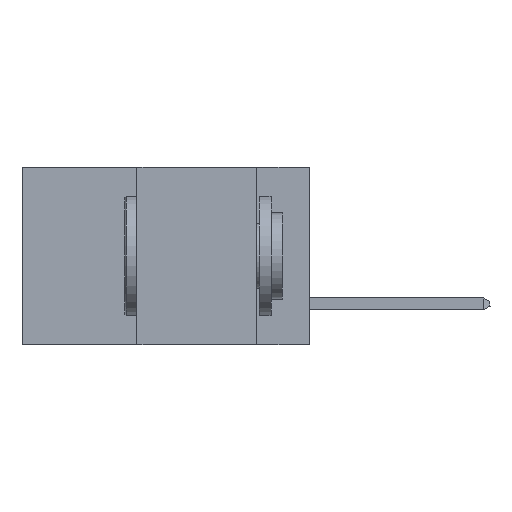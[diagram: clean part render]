
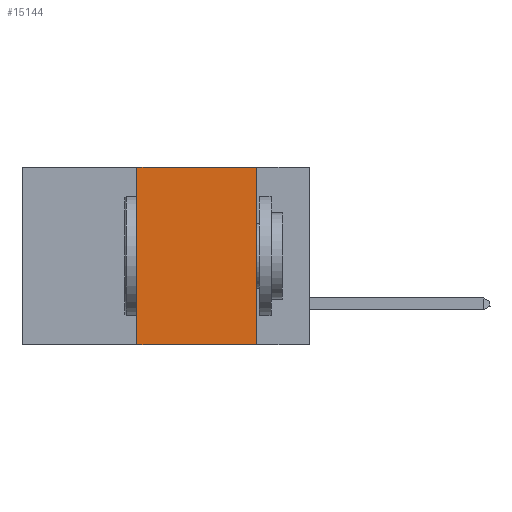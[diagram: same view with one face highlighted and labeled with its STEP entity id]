
A CAD part, left-side view. The second image highlights one B-rep face of the part: STEP entity #15144.
In plain terms, the highlighted planar face has unit normal (-1, 0, 0).
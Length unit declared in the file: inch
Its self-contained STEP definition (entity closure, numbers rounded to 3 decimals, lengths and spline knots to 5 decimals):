
#172 = LINE ( 'NONE', #12849, #17672 ) ;
#372 = CARTESIAN_POINT ( 'NONE',  ( 0., 0.36, 0. ) ) ;
#597 = PLANE ( 'NONE',  #14675 ) ;
#704 = ORIENTED_EDGE ( 'NONE', *, *, #1660, .F. ) ;
#877 = DIRECTION ( 'NONE',  ( 1., 0., 0. ) ) ;
#924 = CARTESIAN_POINT ( 'NONE',  ( 0., 0.11, 0. ) ) ;
#1044 = EDGE_CURVE ( 'NONE', #16447, #6171, #16176, .T. ) ;
#1660 = EDGE_CURVE ( 'NONE', #18354, #16447, #2457, .T. ) ;
#2261 = ORIENTED_EDGE ( 'NONE', *, *, #1044, .F. ) ;
#2457 = LINE ( 'NONE', #10185, #19913 ) ;
#2543 = ORIENTED_EDGE ( 'NONE', *, *, #7121, .T. ) ;
#2648 = CARTESIAN_POINT ( 'NONE',  ( 0., 0.11, -0.37 ) ) ;
#3062 = VERTEX_POINT ( 'NONE', #20383 ) ;
#3455 = DIRECTION ( 'NONE',  ( 0., -1., 0. ) ) ;
#3880 = ORIENTED_EDGE ( 'NONE', *, *, #11488, .F. ) ;
#6171 = VERTEX_POINT ( 'NONE', #2648 ) ;
#7121 = EDGE_CURVE ( 'NONE', #3062, #6171, #14954, .T. ) ;
#8790 = DIRECTION ( 'NONE',  ( 0., 0., 1. ) ) ;
#9815 = FACE_OUTER_BOUND ( 'NONE', #14395, .T. ) ;
#10185 = CARTESIAN_POINT ( 'NONE',  ( 0., 0.6, 0. ) ) ;
#11488 = EDGE_CURVE ( 'NONE', #3062, #18354, #172, .T. ) ;
#12376 = CARTESIAN_POINT ( 'NONE',  ( 0., 0.6, 0. ) ) ;
#12849 = CARTESIAN_POINT ( 'NONE',  ( 0., 0.36, 0. ) ) ;
#13521 = DIRECTION ( 'NONE',  ( 0., -1., 0. ) ) ;
#14395 = EDGE_LOOP ( 'NONE', ( #2261, #704, #3880, #2543 ) ) ;
#14675 = AXIS2_PLACEMENT_3D ( 'NONE', #12376, #877, #16008 ) ;
#14722 = DIRECTION ( 'NONE',  ( 0., 0., -1. ) ) ;
#14954 = LINE ( 'NONE', #18442, #19184 ) ;
#15144 = ADVANCED_FACE ( 'NONE', ( #9815 ), #597, .F. ) ;
#16008 = DIRECTION ( 'NONE',  ( 0., 0., -1. ) ) ;
#16176 = LINE ( 'NONE', #19837, #20377 ) ;
#16447 = VERTEX_POINT ( 'NONE', #924 ) ;
#17672 = VECTOR ( 'NONE', #8790, 39.37008 ) ;
#18354 = VERTEX_POINT ( 'NONE', #372 ) ;
#18442 = CARTESIAN_POINT ( 'NONE',  ( 0., 0.6, -0.37 ) ) ;
#19184 = VECTOR ( 'NONE', #13521, 39.37008 ) ;
#19837 = CARTESIAN_POINT ( 'NONE',  ( 0., 0.11, 0. ) ) ;
#19913 = VECTOR ( 'NONE', #3455, 39.37008 ) ;
#20377 = VECTOR ( 'NONE', #14722, 39.37008 ) ;
#20383 = CARTESIAN_POINT ( 'NONE',  ( 0., 0.36, -0.37 ) ) ;
